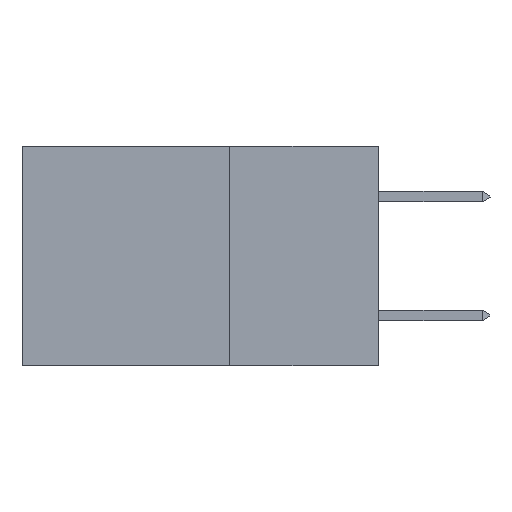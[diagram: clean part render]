
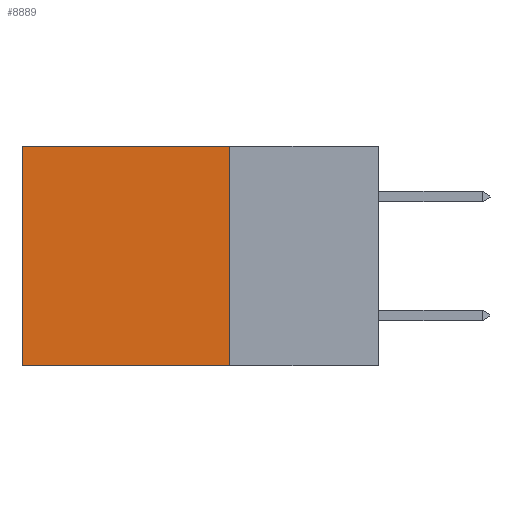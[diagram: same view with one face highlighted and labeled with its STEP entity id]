
A CAD part, left-side view. The second image highlights one B-rep face of the part: STEP entity #8889.
In plain terms, the highlighted planar face has unit normal (-1, 0, 0).
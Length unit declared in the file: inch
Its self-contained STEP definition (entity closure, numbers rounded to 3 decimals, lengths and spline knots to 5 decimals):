
#457 = CARTESIAN_POINT ( 'NONE',  ( 0.298, 0.25, -0.37 ) ) ;
#553 = DIRECTION ( 'NONE',  ( 0., 1., 0. ) ) ;
#692 = LINE ( 'NONE', #14872, #1411 ) ;
#1411 = VECTOR ( 'NONE', #23757, 39.37008 ) ;
#2771 = CARTESIAN_POINT ( 'NONE',  ( 0.298, 0.25, 0. ) ) ;
#3076 = CARTESIAN_POINT ( 'NONE',  ( 0.298, 0.6, 0. ) ) ;
#3880 = CARTESIAN_POINT ( 'NONE',  ( 0.298, 0.25, 0. ) ) ;
#3998 = CARTESIAN_POINT ( 'NONE',  ( 0.298, 0.25, 0. ) ) ;
#4433 = CARTESIAN_POINT ( 'NONE',  ( 0.298, 0.25, 0. ) ) ;
#6765 = DIRECTION ( 'NONE',  ( 0., 0., -1. ) ) ;
#6967 = ORIENTED_EDGE ( 'NONE', *, *, #29877, .F. ) ;
#7009 = LINE ( 'NONE', #4433, #12456 ) ;
#7917 = VECTOR ( 'NONE', #27136, 39.37008 ) ;
#8889 = ADVANCED_FACE ( 'NONE', ( #24302 ), #27005, .F. ) ;
#10230 = EDGE_CURVE ( 'NONE', #27696, #20856, #692, .T. ) ;
#12456 = VECTOR ( 'NONE', #6765, 39.37008 ) ;
#13123 = DIRECTION ( 'NONE',  ( 0., 0., -1. ) ) ;
#13367 = VERTEX_POINT ( 'NONE', #457 ) ;
#14105 = LINE ( 'NONE', #24777, #7917 ) ;
#14872 = CARTESIAN_POINT ( 'NONE',  ( 0.298, 0.6, 0. ) ) ;
#16623 = VECTOR ( 'NONE', #553, 39.37008 ) ;
#17468 = VERTEX_POINT ( 'NONE', #3998 ) ;
#20177 = CARTESIAN_POINT ( 'NONE',  ( 0.298, 0.6, -0.37 ) ) ;
#20856 = VERTEX_POINT ( 'NONE', #20177 ) ;
#22411 = ORIENTED_EDGE ( 'NONE', *, *, #27470, .F. ) ;
#23089 = AXIS2_PLACEMENT_3D ( 'NONE', #3880, #24740, #13123 ) ;
#23563 = ORIENTED_EDGE ( 'NONE', *, *, #10230, .T. ) ;
#23757 = DIRECTION ( 'NONE',  ( 0., 0., -1. ) ) ;
#24302 = FACE_OUTER_BOUND ( 'NONE', #27533, .T. ) ;
#24740 = DIRECTION ( 'NONE',  ( 1., 0., 0. ) ) ;
#24777 = CARTESIAN_POINT ( 'NONE',  ( 0.298, 0.25, -0.37 ) ) ;
#27005 = PLANE ( 'NONE',  #23089 ) ;
#27007 = EDGE_CURVE ( 'NONE', #17468, #27696, #28962, .T. ) ;
#27136 = DIRECTION ( 'NONE',  ( 0., 1., 0. ) ) ;
#27470 = EDGE_CURVE ( 'NONE', #13367, #20856, #14105, .T. ) ;
#27533 = EDGE_LOOP ( 'NONE', ( #23563, #22411, #6967, #29785 ) ) ;
#27696 = VERTEX_POINT ( 'NONE', #3076 ) ;
#28962 = LINE ( 'NONE', #2771, #16623 ) ;
#29785 = ORIENTED_EDGE ( 'NONE', *, *, #27007, .T. ) ;
#29877 = EDGE_CURVE ( 'NONE', #17468, #13367, #7009, .T. ) ;
